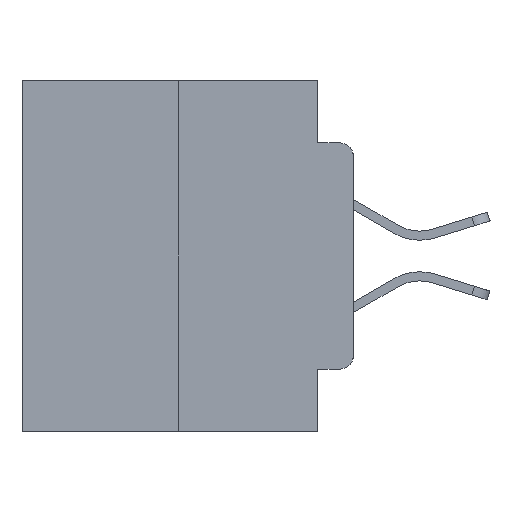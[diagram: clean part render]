
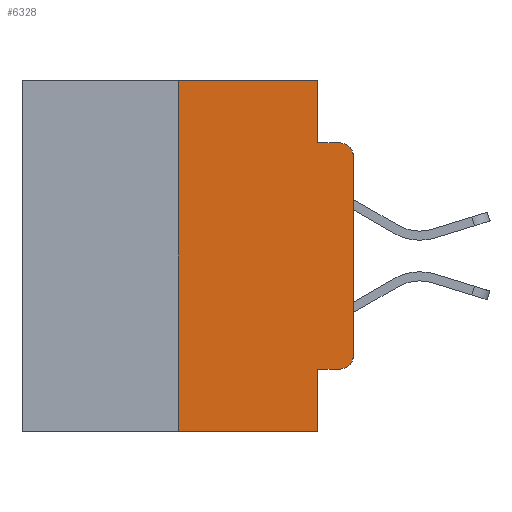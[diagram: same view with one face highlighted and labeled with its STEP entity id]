
A CAD part, left-side view. The second image highlights one B-rep face of the part: STEP entity #6328.
In plain terms, the highlighted planar face has unit normal (-1, 0, 0).
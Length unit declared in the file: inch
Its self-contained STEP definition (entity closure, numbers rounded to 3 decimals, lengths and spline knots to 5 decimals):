
#2 = EDGE_CURVE ( 'NONE', #5531, #7704, #2120, .T. ) ;
#195 = LINE ( 'NONE', #12136, #1583 ) ;
#202 = LINE ( 'NONE', #218, #16725 ) ;
#218 = CARTESIAN_POINT ( 'NONE',  ( 0., 0.051, 0. ) ) ;
#304 = ORIENTED_EDGE ( 'NONE', *, *, #18736, .F. ) ;
#678 = LINE ( 'NONE', #23741, #22689 ) ;
#829 = VECTOR ( 'NONE', #4006, 39.37008 ) ;
#1583 = VECTOR ( 'NONE', #26766, 39.37008 ) ;
#2120 = LINE ( 'NONE', #26300, #24086 ) ;
#3025 = ORIENTED_EDGE ( 'NONE', *, *, #27499, .T. ) ;
#3281 = CIRCLE ( 'NONE', #13508, 0.02 ) ;
#4006 = DIRECTION ( 'NONE',  ( 0., 0., 1. ) ) ;
#4530 = CARTESIAN_POINT ( 'NONE',  ( 0., 0.051, -0.4115 ) ) ;
#5287 = VERTEX_POINT ( 'NONE', #6063 ) ;
#5531 = VERTEX_POINT ( 'NONE', #23815 ) ;
#6063 = CARTESIAN_POINT ( 'NONE',  ( 0., 0.02, -0.4115 ) ) ;
#6328 = ADVANCED_FACE ( 'NONE', ( #22338 ), #24223, .F. ) ;
#6611 = LINE ( 'NONE', #23047, #829 ) ;
#6673 = VECTOR ( 'NONE', #15944, 39.37008 ) ;
#6785 = ORIENTED_EDGE ( 'NONE', *, *, #22645, .F. ) ;
#7152 = LINE ( 'NONE', #4530, #23355 ) ;
#7559 = CARTESIAN_POINT ( 'NONE',  ( 0., 0.25, 0. ) ) ;
#7704 = VERTEX_POINT ( 'NONE', #26856 ) ;
#7715 = DIRECTION ( 'NONE',  ( -1., 0., 0. ) ) ;
#8632 = EDGE_LOOP ( 'NONE', ( #25610, #3025, #24265, #10956, #6785, #304, #19309, #11783, #23965, #14181 ) ) ;
#9500 = CARTESIAN_POINT ( 'NONE',  ( 0., 0.473, 0. ) ) ;
#10125 = DIRECTION ( 'NONE',  ( -1., 0., 0. ) ) ;
#10956 = ORIENTED_EDGE ( 'NONE', *, *, #15633, .F. ) ;
#11181 = EDGE_CURVE ( 'NONE', #16447, #7704, #22893, .T. ) ;
#11247 = VECTOR ( 'NONE', #18360, 39.37008 ) ;
#11783 = ORIENTED_EDGE ( 'NONE', *, *, #2, .F. ) ;
#12136 = CARTESIAN_POINT ( 'NONE',  ( 0., 0.473, 0. ) ) ;
#12416 = VERTEX_POINT ( 'NONE', #7559 ) ;
#13508 = AXIS2_PLACEMENT_3D ( 'NONE', #22731, #10125, #24836 ) ;
#13796 = DIRECTION ( 'NONE',  ( 0., 0., -1. ) ) ;
#14119 = CARTESIAN_POINT ( 'NONE',  ( 0., 0.051, -0.0885 ) ) ;
#14181 = ORIENTED_EDGE ( 'NONE', *, *, #16475, .T. ) ;
#15251 = CARTESIAN_POINT ( 'NONE',  ( 0., 0., -0.1085 ) ) ;
#15446 = DIRECTION ( 'NONE',  ( 0., -1., 0. ) ) ;
#15633 = EDGE_CURVE ( 'NONE', #23943, #15888, #202, .T. ) ;
#15833 = VERTEX_POINT ( 'NONE', #15974 ) ;
#15888 = VERTEX_POINT ( 'NONE', #14119 ) ;
#15944 = DIRECTION ( 'NONE',  ( 0., -1., 0. ) ) ;
#15974 = CARTESIAN_POINT ( 'NONE',  ( 0., 0.02, -0.0885 ) ) ;
#16447 = VERTEX_POINT ( 'NONE', #18218 ) ;
#16475 = EDGE_CURVE ( 'NONE', #5287, #23536, #23525, .T. ) ;
#16725 = VECTOR ( 'NONE', #19623, 39.37008 ) ;
#17928 = AXIS2_PLACEMENT_3D ( 'NONE', #9500, #26296, #13796 ) ;
#17934 = AXIS2_PLACEMENT_3D ( 'NONE', #20405, #7715, #22488 ) ;
#18051 = DIRECTION ( 'NONE',  ( 0., 0., -1. ) ) ;
#18218 = CARTESIAN_POINT ( 'NONE',  ( 0., 0.25, -0.5 ) ) ;
#18360 = DIRECTION ( 'NONE',  ( 0., 0., 1. ) ) ;
#18736 = EDGE_CURVE ( 'NONE', #16447, #12416, #23100, .T. ) ;
#19309 = ORIENTED_EDGE ( 'NONE', *, *, #11181, .T. ) ;
#19623 = DIRECTION ( 'NONE',  ( 0., 0., -1. ) ) ;
#20405 = CARTESIAN_POINT ( 'NONE',  ( 0., 0.02, -0.3915 ) ) ;
#20639 = VERTEX_POINT ( 'NONE', #15251 ) ;
#20657 = EDGE_CURVE ( 'NONE', #5531, #5287, #7152, .T. ) ;
#20689 = EDGE_CURVE ( 'NONE', #15888, #15833, #678, .T. ) ;
#22137 = CARTESIAN_POINT ( 'NONE',  ( 0., 0.473, -0.5 ) ) ;
#22338 = FACE_OUTER_BOUND ( 'NONE', #8632, .T. ) ;
#22445 = CARTESIAN_POINT ( 'NONE',  ( 0., 0.25, 0. ) ) ;
#22488 = DIRECTION ( 'NONE',  ( 0., 0., -1. ) ) ;
#22645 = EDGE_CURVE ( 'NONE', #12416, #23943, #195, .T. ) ;
#22689 = VECTOR ( 'NONE', #15446, 39.37008 ) ;
#22731 = CARTESIAN_POINT ( 'NONE',  ( 0., 0.02, -0.1085 ) ) ;
#22893 = LINE ( 'NONE', #22137, #6673 ) ;
#23047 = CARTESIAN_POINT ( 'NONE',  ( 0., 0., 0. ) ) ;
#23100 = LINE ( 'NONE', #22445, #11247 ) ;
#23355 = VECTOR ( 'NONE', #23653, 39.37008 ) ;
#23525 = CIRCLE ( 'NONE', #17934, 0.02 ) ;
#23536 = VERTEX_POINT ( 'NONE', #27337 ) ;
#23653 = DIRECTION ( 'NONE',  ( 0., -1., 0. ) ) ;
#23741 = CARTESIAN_POINT ( 'NONE',  ( 0., 0.051, -0.0885 ) ) ;
#23815 = CARTESIAN_POINT ( 'NONE',  ( 0., 0.051, -0.4115 ) ) ;
#23943 = VERTEX_POINT ( 'NONE', #25094 ) ;
#23965 = ORIENTED_EDGE ( 'NONE', *, *, #20657, .T. ) ;
#24086 = VECTOR ( 'NONE', #18051, 39.37008 ) ;
#24223 = PLANE ( 'NONE',  #17928 ) ;
#24265 = ORIENTED_EDGE ( 'NONE', *, *, #20689, .F. ) ;
#24609 = EDGE_CURVE ( 'NONE', #23536, #20639, #6611, .T. ) ;
#24836 = DIRECTION ( 'NONE',  ( 0., 0., -1. ) ) ;
#25094 = CARTESIAN_POINT ( 'NONE',  ( 0., 0.051, 0. ) ) ;
#25610 = ORIENTED_EDGE ( 'NONE', *, *, #24609, .T. ) ;
#26296 = DIRECTION ( 'NONE',  ( 1., 0., 0. ) ) ;
#26300 = CARTESIAN_POINT ( 'NONE',  ( 0., 0.051, 0. ) ) ;
#26766 = DIRECTION ( 'NONE',  ( 0., -1., 0. ) ) ;
#26856 = CARTESIAN_POINT ( 'NONE',  ( 0., 0.051, -0.5 ) ) ;
#27337 = CARTESIAN_POINT ( 'NONE',  ( 0., 0., -0.3915 ) ) ;
#27499 = EDGE_CURVE ( 'NONE', #20639, #15833, #3281, .T. ) ;
